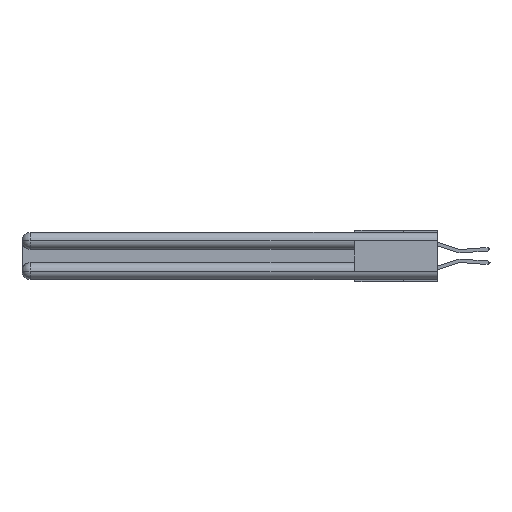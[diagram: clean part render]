
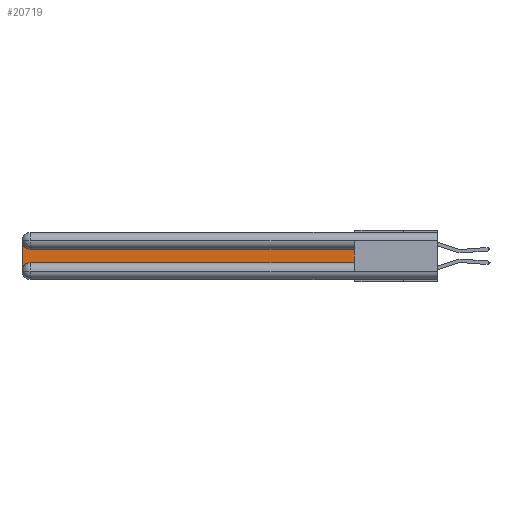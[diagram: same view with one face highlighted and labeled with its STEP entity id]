
A CAD part, left-side view. The second image highlights one B-rep face of the part: STEP entity #20719.
In plain terms, the highlighted planar face has unit normal (-1, 0, 0).
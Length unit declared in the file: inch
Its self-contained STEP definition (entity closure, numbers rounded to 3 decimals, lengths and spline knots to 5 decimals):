
#39 = DIRECTION ( 'NONE',  ( 1., 0., 0. ) ) ;
#1073 = ORIENTED_EDGE ( 'NONE', *, *, #11409, .T. ) ;
#1105 = LINE ( 'NONE', #17150, #26365 ) ;
#1564 = ORIENTED_EDGE ( 'NONE', *, *, #4062, .T. ) ;
#3181 = DIRECTION ( 'NONE',  ( 1., 0., 0. ) ) ;
#3400 = EDGE_LOOP ( 'NONE', ( #1073, #15604, #5743, #1564, #4111, #15485 ) ) ;
#4062 = EDGE_CURVE ( 'NONE', #11263, #11177, #29293, .T. ) ;
#4111 = ORIENTED_EDGE ( 'NONE', *, *, #13377, .T. ) ;
#5743 = ORIENTED_EDGE ( 'NONE', *, *, #7730, .T. ) ;
#6313 = CARTESIAN_POINT ( 'NONE',  ( 0.075, 3., -0.0625 ) ) ;
#6693 = DIRECTION ( 'NONE',  ( 0., 0., -1. ) ) ;
#6724 = DIRECTION ( 'NONE',  ( 0., 0., 1. ) ) ;
#7730 = EDGE_CURVE ( 'NONE', #18657, #11263, #24621, .T. ) ;
#8893 = VERTEX_POINT ( 'NONE', #21285 ) ;
#9406 = CARTESIAN_POINT ( 'NONE',  ( 0.075, 2.94, -0.1225 ) ) ;
#9530 = CARTESIAN_POINT ( 'NONE',  ( 0.075, 2.94, -0.2175 ) ) ;
#9939 = DIRECTION ( 'NONE',  ( 0., 1., 0. ) ) ;
#10003 = VERTEX_POINT ( 'NONE', #9406 ) ;
#10137 = CARTESIAN_POINT ( 'NONE',  ( 0.075, 2.94, -0.2775 ) ) ;
#10182 = AXIS2_PLACEMENT_3D ( 'NONE', #10137, #3181, #19771 ) ;
#11135 = FACE_OUTER_BOUND ( 'NONE', #3400, .T. ) ;
#11177 = VERTEX_POINT ( 'NONE', #9530 ) ;
#11263 = VERTEX_POINT ( 'NONE', #28435 ) ;
#11409 = EDGE_CURVE ( 'NONE', #8893, #10003, #1105, .T. ) ;
#12726 = PLANE ( 'NONE',  #26017 ) ;
#13377 = EDGE_CURVE ( 'NONE', #11177, #14200, #21833, .T. ) ;
#13465 = CARTESIAN_POINT ( 'NONE',  ( 0.075, 0.6, -0.2175 ) ) ;
#14200 = VERTEX_POINT ( 'NONE', #29981 ) ;
#14288 = CARTESIAN_POINT ( 'NONE',  ( 0.075, 2.94, -0.0625 ) ) ;
#15485 = ORIENTED_EDGE ( 'NONE', *, *, #28480, .T. ) ;
#15604 = ORIENTED_EDGE ( 'NONE', *, *, #22500, .T. ) ;
#15932 = CARTESIAN_POINT ( 'NONE',  ( 0.075, 3., -0.2175 ) ) ;
#17043 = CIRCLE ( 'NONE', #29044, 0.06 ) ;
#17150 = CARTESIAN_POINT ( 'NONE',  ( 0.075, 0.6, -0.1225 ) ) ;
#17479 = CARTESIAN_POINT ( 'NONE',  ( 0.075, 3., -0.1225 ) ) ;
#18657 = VERTEX_POINT ( 'NONE', #6313 ) ;
#19043 = DIRECTION ( 'NONE',  ( 0., 0., -1. ) ) ;
#19540 = VECTOR ( 'NONE', #29842, 39.37008 ) ;
#19672 = DIRECTION ( 'NONE',  ( 0., 0., -1. ) ) ;
#19771 = DIRECTION ( 'NONE',  ( 0., 0., -1. ) ) ;
#20719 = ADVANCED_FACE ( 'NONE', ( #11135 ), #12726, .F. ) ;
#21285 = CARTESIAN_POINT ( 'NONE',  ( 0.075, 0.6, -0.1225 ) ) ;
#21833 = LINE ( 'NONE', #13465, #19540 ) ;
#22500 = EDGE_CURVE ( 'NONE', #10003, #18657, #17043, .T. ) ;
#23894 = VECTOR ( 'NONE', #6724, 39.37008 ) ;
#24288 = LINE ( 'NONE', #25638, #23894 ) ;
#24621 = LINE ( 'NONE', #15932, #26826 ) ;
#25638 = CARTESIAN_POINT ( 'NONE',  ( 0.075, 0.6, -0.2175 ) ) ;
#26017 = AXIS2_PLACEMENT_3D ( 'NONE', #17479, #26867, #19672 ) ;
#26365 = VECTOR ( 'NONE', #9939, 39.37008 ) ;
#26826 = VECTOR ( 'NONE', #6693, 39.37008 ) ;
#26867 = DIRECTION ( 'NONE',  ( 1., 0., 0. ) ) ;
#28435 = CARTESIAN_POINT ( 'NONE',  ( 0.075, 3., -0.2775 ) ) ;
#28480 = EDGE_CURVE ( 'NONE', #14200, #8893, #24288, .T. ) ;
#29044 = AXIS2_PLACEMENT_3D ( 'NONE', #14288, #39, #19043 ) ;
#29293 = CIRCLE ( 'NONE', #10182, 0.06 ) ;
#29842 = DIRECTION ( 'NONE',  ( 0., -1., 0. ) ) ;
#29981 = CARTESIAN_POINT ( 'NONE',  ( 0.075, 0.6, -0.2175 ) ) ;
